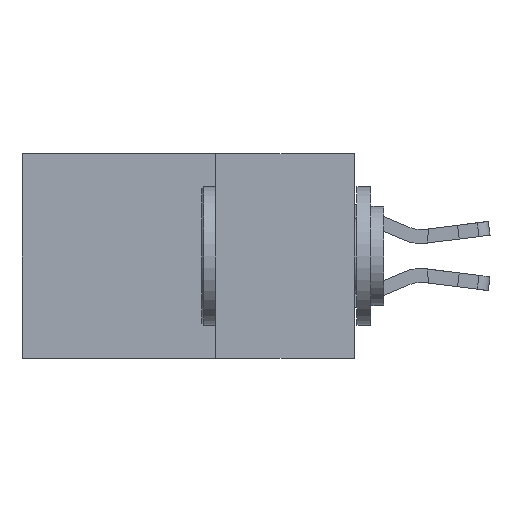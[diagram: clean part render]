
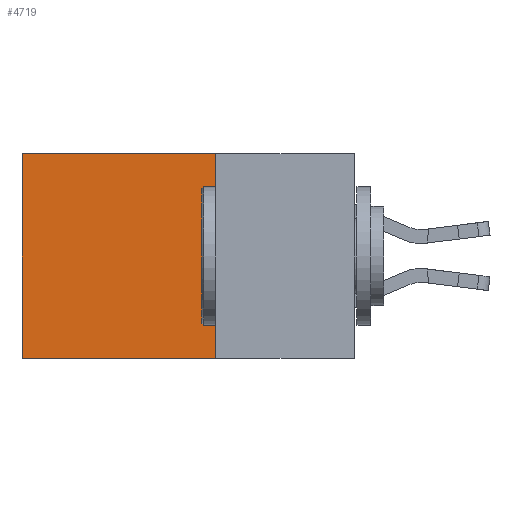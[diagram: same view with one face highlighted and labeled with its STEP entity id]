
A CAD part, left-side view. The second image highlights one B-rep face of the part: STEP entity #4719.
In plain terms, the highlighted planar face has unit normal (-1, 0, 0).
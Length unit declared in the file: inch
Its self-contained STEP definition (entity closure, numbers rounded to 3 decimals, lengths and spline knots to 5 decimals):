
#221 = VECTOR ( 'NONE', #4752, 39.37008 ) ;
#289 = VERTEX_POINT ( 'NONE', #13078 ) ;
#1435 = EDGE_CURVE ( 'NONE', #12691, #6724, #1650, .T. ) ;
#1650 = LINE ( 'NONE', #10906, #221 ) ;
#1909 = CARTESIAN_POINT ( 'NONE',  ( 0.2615, 0.25, -0.37 ) ) ;
#2157 = DIRECTION ( 'NONE',  ( 0., 0., -1. ) ) ;
#2488 = ORIENTED_EDGE ( 'NONE', *, *, #2757, .F. ) ;
#2757 = EDGE_CURVE ( 'NONE', #11271, #289, #13323, .T. ) ;
#3147 = CARTESIAN_POINT ( 'NONE',  ( 0.2615, 0.6, -0.37 ) ) ;
#3716 = DIRECTION ( 'NONE',  ( 0., 0., -1. ) ) ;
#3982 = ORIENTED_EDGE ( 'NONE', *, *, #1435, .T. ) ;
#4172 = DIRECTION ( 'NONE',  ( 0., 1., 0. ) ) ;
#4304 = EDGE_LOOP ( 'NONE', ( #3982, #7237, #2488, #8765 ) ) ;
#4685 = EDGE_CURVE ( 'NONE', #11271, #12691, #11495, .T. ) ;
#4719 = ADVANCED_FACE ( 'NONE', ( #10534 ), #5561, .F. ) ;
#4723 = CARTESIAN_POINT ( 'NONE',  ( 0.2615, 0.25, 0. ) ) ;
#4752 = DIRECTION ( 'NONE',  ( 0., 0., -1. ) ) ;
#5561 = PLANE ( 'NONE',  #9223 ) ;
#6200 = VECTOR ( 'NONE', #10345, 39.37008 ) ;
#6724 = VERTEX_POINT ( 'NONE', #3147 ) ;
#6848 = CARTESIAN_POINT ( 'NONE',  ( 0.2615, 0.25, -0.37 ) ) ;
#7237 = ORIENTED_EDGE ( 'NONE', *, *, #11775, .F. ) ;
#7451 = CARTESIAN_POINT ( 'NONE',  ( 0.2615, 0.6, 0. ) ) ;
#8746 = CARTESIAN_POINT ( 'NONE',  ( 0.2615, 0.25, -0.37 ) ) ;
#8765 = ORIENTED_EDGE ( 'NONE', *, *, #4685, .T. ) ;
#9223 = AXIS2_PLACEMENT_3D ( 'NONE', #8746, #10808, #2157 ) ;
#10345 = DIRECTION ( 'NONE',  ( 0., 1., 0. ) ) ;
#10534 = FACE_OUTER_BOUND ( 'NONE', #4304, .T. ) ;
#10808 = DIRECTION ( 'NONE',  ( 1., 0., 0. ) ) ;
#10906 = CARTESIAN_POINT ( 'NONE',  ( 0.2615, 0.6, -0.37 ) ) ;
#11259 = CARTESIAN_POINT ( 'NONE',  ( 0.2615, 0.25, 0. ) ) ;
#11271 = VERTEX_POINT ( 'NONE', #11259 ) ;
#11495 = LINE ( 'NONE', #4723, #12727 ) ;
#11712 = VECTOR ( 'NONE', #3716, 39.37008 ) ;
#11775 = EDGE_CURVE ( 'NONE', #289, #6724, #12279, .T. ) ;
#12279 = LINE ( 'NONE', #1909, #6200 ) ;
#12691 = VERTEX_POINT ( 'NONE', #7451 ) ;
#12727 = VECTOR ( 'NONE', #4172, 39.37008 ) ;
#13078 = CARTESIAN_POINT ( 'NONE',  ( 0.2615, 0.25, -0.37 ) ) ;
#13323 = LINE ( 'NONE', #6848, #11712 ) ;
